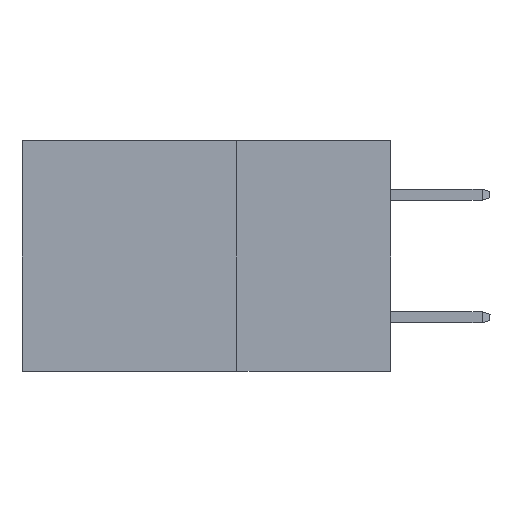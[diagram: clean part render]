
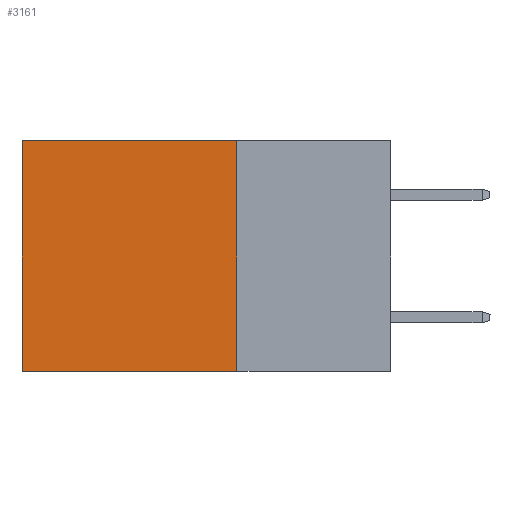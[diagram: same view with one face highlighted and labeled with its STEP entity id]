
A CAD part, left-side view. The second image highlights one B-rep face of the part: STEP entity #3161.
In plain terms, the highlighted planar face has unit normal (-1, 0, 0).
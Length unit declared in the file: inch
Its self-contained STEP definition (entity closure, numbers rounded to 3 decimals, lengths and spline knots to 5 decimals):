
#149 = VERTEX_POINT ( 'NONE', #15316 ) ;
#721 = ORIENTED_EDGE ( 'NONE', *, *, #5916, .F. ) ;
#844 = ORIENTED_EDGE ( 'NONE', *, *, #7934, .T. ) ;
#868 = LINE ( 'NONE', #11822, #2967 ) ;
#1606 = CARTESIAN_POINT ( 'NONE',  ( 0.2875, 0.25, 0. ) ) ;
#1700 = PLANE ( 'NONE',  #13592 ) ;
#2222 = VECTOR ( 'NONE', #15269, 39.37008 ) ;
#2720 = VECTOR ( 'NONE', #15739, 39.37008 ) ;
#2759 = ORIENTED_EDGE ( 'NONE', *, *, #13925, .F. ) ;
#2967 = VECTOR ( 'NONE', #14366, 39.37008 ) ;
#3018 = CARTESIAN_POINT ( 'NONE',  ( 0.2875, 0.25, -0.375 ) ) ;
#3161 = ADVANCED_FACE ( 'NONE', ( #5646 ), #1700, .F. ) ;
#3468 = VERTEX_POINT ( 'NONE', #1606 ) ;
#4114 = VERTEX_POINT ( 'NONE', #6959 ) ;
#5169 = DIRECTION ( 'NONE',  ( 0., 0., -1. ) ) ;
#5646 = FACE_OUTER_BOUND ( 'NONE', #11362, .T. ) ;
#5916 = EDGE_CURVE ( 'NONE', #3468, #12688, #15247, .T. ) ;
#6448 = DIRECTION ( 'NONE',  ( 1., 0., 0. ) ) ;
#6959 = CARTESIAN_POINT ( 'NONE',  ( 0.2875, 0.6, -0.375 ) ) ;
#7028 = VECTOR ( 'NONE', #9100, 39.37008 ) ;
#7655 = LINE ( 'NONE', #8142, #2720 ) ;
#7934 = EDGE_CURVE ( 'NONE', #149, #4114, #868, .T. ) ;
#8142 = CARTESIAN_POINT ( 'NONE',  ( 0.2875, 0.25, 0. ) ) ;
#8810 = CARTESIAN_POINT ( 'NONE',  ( 0.2875, 0.25, -0.375 ) ) ;
#9100 = DIRECTION ( 'NONE',  ( 0., 0., -1. ) ) ;
#10064 = EDGE_CURVE ( 'NONE', #3468, #149, #7655, .T. ) ;
#11252 = CARTESIAN_POINT ( 'NONE',  ( 0.2875, 0.25, -0.375 ) ) ;
#11362 = EDGE_LOOP ( 'NONE', ( #844, #2759, #721, #11786 ) ) ;
#11786 = ORIENTED_EDGE ( 'NONE', *, *, #10064, .T. ) ;
#11822 = CARTESIAN_POINT ( 'NONE',  ( 0.2875, 0.6, -0.375 ) ) ;
#12688 = VERTEX_POINT ( 'NONE', #8810 ) ;
#13592 = AXIS2_PLACEMENT_3D ( 'NONE', #11252, #6448, #5169 ) ;
#13644 = LINE ( 'NONE', #14067, #2222 ) ;
#13925 = EDGE_CURVE ( 'NONE', #12688, #4114, #13644, .T. ) ;
#14067 = CARTESIAN_POINT ( 'NONE',  ( 0.2875, 0.25, -0.375 ) ) ;
#14366 = DIRECTION ( 'NONE',  ( 0., 0., -1. ) ) ;
#15247 = LINE ( 'NONE', #3018, #7028 ) ;
#15269 = DIRECTION ( 'NONE',  ( 0., 1., 0. ) ) ;
#15316 = CARTESIAN_POINT ( 'NONE',  ( 0.2875, 0.6, 0. ) ) ;
#15739 = DIRECTION ( 'NONE',  ( 0., 1., 0. ) ) ;
